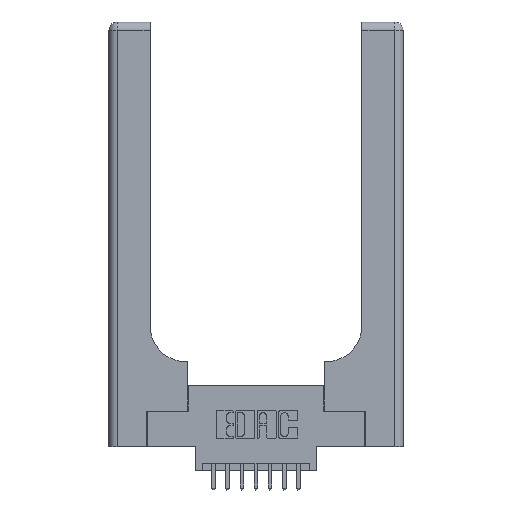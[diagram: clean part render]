
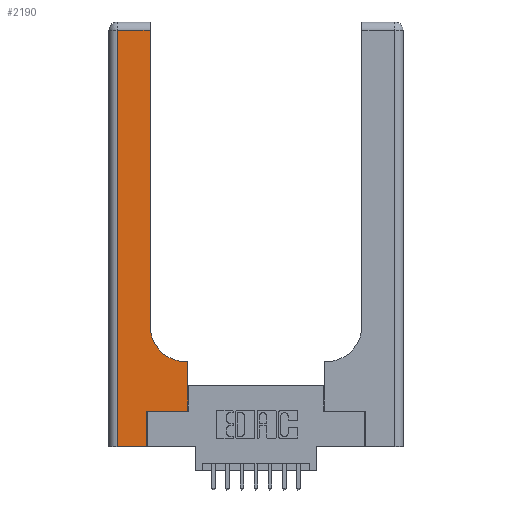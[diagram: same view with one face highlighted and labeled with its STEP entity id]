
A CAD part, top view. The second image highlights one B-rep face of the part: STEP entity #2190.
In plain terms, the highlighted planar face has unit normal (0, 0, 1).
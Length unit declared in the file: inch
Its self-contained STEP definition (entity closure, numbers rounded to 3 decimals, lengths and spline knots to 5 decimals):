
#70 = CARTESIAN_POINT ( 'NONE',  ( 0., 2.94, 0.37 ) ) ;
#260 = EDGE_CURVE ( 'NONE', #14906, #10242, #384, .T. ) ;
#367 = DIRECTION ( 'NONE',  ( -1., 0., 0. ) ) ;
#384 = LINE ( 'NONE', #7655, #14273 ) ;
#699 = CARTESIAN_POINT ( 'NONE',  ( 0.2915, 0.85, 0.37 ) ) ;
#1357 = VERTEX_POINT ( 'NONE', #14289 ) ;
#1389 = DIRECTION ( 'NONE',  ( 1., 0., 0. ) ) ;
#1501 = VERTEX_POINT ( 'NONE', #14553 ) ;
#1813 = DIRECTION ( 'NONE',  ( 0., -1., 0. ) ) ;
#1826 = EDGE_LOOP ( 'NONE', ( #10943, #7124, #8172, #3661, #12264, #11714, #10814, #2758, #12633 ) ) ;
#1890 = VERTEX_POINT ( 'NONE', #3290 ) ;
#2190 = ADVANCED_FACE ( 'NONE', ( #2888 ), #12406, .F. ) ;
#2295 = AXIS2_PLACEMENT_3D ( 'NONE', #10333, #4394, #4304 ) ;
#2758 = ORIENTED_EDGE ( 'NONE', *, *, #260, .T. ) ;
#2888 = FACE_OUTER_BOUND ( 'NONE', #1826, .T. ) ;
#3202 = DIRECTION ( 'NONE',  ( -1., 0., 0. ) ) ;
#3290 = CARTESIAN_POINT ( 'NONE',  ( 0.06, 0., 0.37 ) ) ;
#3437 = VERTEX_POINT ( 'NONE', #9979 ) ;
#3661 = ORIENTED_EDGE ( 'NONE', *, *, #9320, .T. ) ;
#3778 = EDGE_CURVE ( 'NONE', #10242, #10791, #13706, .T. ) ;
#3946 = EDGE_CURVE ( 'NONE', #1501, #14906, #14652, .T. ) ;
#4304 = DIRECTION ( 'NONE',  ( 1., 0., 0. ) ) ;
#4394 = DIRECTION ( 'NONE',  ( 0., 0., -1. ) ) ;
#4674 = LINE ( 'NONE', #9700, #7857 ) ;
#4717 = CARTESIAN_POINT ( 'NONE',  ( 0.5585, 0.6, 0.37 ) ) ;
#4750 = LINE ( 'NONE', #70, #8299 ) ;
#5001 = CARTESIAN_POINT ( 'NONE',  ( 0.269, 0.25, 0.37 ) ) ;
#5084 = CARTESIAN_POINT ( 'NONE',  ( 0.269, 0.25, 0.37 ) ) ;
#5928 = VERTEX_POINT ( 'NONE', #6114 ) ;
#6114 = CARTESIAN_POINT ( 'NONE',  ( 0.2915, 2.94, 0.37 ) ) ;
#6499 = EDGE_CURVE ( 'NONE', #5928, #3437, #4750, .T. ) ;
#6683 = VECTOR ( 'NONE', #14177, 39.37008 ) ;
#6709 = VECTOR ( 'NONE', #1813, 39.37008 ) ;
#6861 = VECTOR ( 'NONE', #12170, 39.37008 ) ;
#7124 = ORIENTED_EDGE ( 'NONE', *, *, #6499, .T. ) ;
#7655 = CARTESIAN_POINT ( 'NONE',  ( 0.2915, 0.6, 0.37 ) ) ;
#7807 = LINE ( 'NONE', #10954, #6861 ) ;
#7857 = VECTOR ( 'NONE', #12146, 39.37008 ) ;
#7888 = EDGE_CURVE ( 'NONE', #1357, #15262, #8619, .T. ) ;
#8172 = ORIENTED_EDGE ( 'NONE', *, *, #10016, .T. ) ;
#8299 = VECTOR ( 'NONE', #13073, 39.37008 ) ;
#8619 = LINE ( 'NONE', #10103, #11353 ) ;
#9311 = VECTOR ( 'NONE', #1389, 39.37008 ) ;
#9320 = EDGE_CURVE ( 'NONE', #1890, #1357, #4674, .T. ) ;
#9700 = CARTESIAN_POINT ( 'NONE',  ( 0., 0., 0.37 ) ) ;
#9979 = CARTESIAN_POINT ( 'NONE',  ( 0.06, 2.94, 0.37 ) ) ;
#10016 = EDGE_CURVE ( 'NONE', #3437, #1890, #13537, .T. ) ;
#10076 = DIRECTION ( 'NONE',  ( 0., 0., -1. ) ) ;
#10103 = CARTESIAN_POINT ( 'NONE',  ( 0.269, 0., 0.37 ) ) ;
#10242 = VERTEX_POINT ( 'NONE', #14617 ) ;
#10333 = CARTESIAN_POINT ( 'NONE',  ( 0.5415, 0.85, 0.37 ) ) ;
#10791 = VERTEX_POINT ( 'NONE', #699 ) ;
#10814 = ORIENTED_EDGE ( 'NONE', *, *, #3946, .T. ) ;
#10943 = ORIENTED_EDGE ( 'NONE', *, *, #15510, .T. ) ;
#10954 = CARTESIAN_POINT ( 'NONE',  ( 0.2915, 3., 0.37 ) ) ;
#11353 = VECTOR ( 'NONE', #14879, 39.37008 ) ;
#11714 = ORIENTED_EDGE ( 'NONE', *, *, #15156, .T. ) ;
#12146 = DIRECTION ( 'NONE',  ( 1., 0., 0. ) ) ;
#12170 = DIRECTION ( 'NONE',  ( 0., 1., 0. ) ) ;
#12264 = ORIENTED_EDGE ( 'NONE', *, *, #7888, .T. ) ;
#12406 = PLANE ( 'NONE',  #13858 ) ;
#12633 = ORIENTED_EDGE ( 'NONE', *, *, #3778, .T. ) ;
#12811 = CARTESIAN_POINT ( 'NONE',  ( 0.06, 3., 0.37 ) ) ;
#12957 = CARTESIAN_POINT ( 'NONE',  ( 0.5585, 0.25, 0.37 ) ) ;
#13073 = DIRECTION ( 'NONE',  ( -1., 0., 0. ) ) ;
#13537 = LINE ( 'NONE', #12811, #6709 ) ;
#13626 = CARTESIAN_POINT ( 'NONE',  ( 0., 3., 0.37 ) ) ;
#13706 = CIRCLE ( 'NONE', #2295, 0.25 ) ;
#13858 = AXIS2_PLACEMENT_3D ( 'NONE', #13626, #10076, #367 ) ;
#14177 = DIRECTION ( 'NONE',  ( 0., 1., 0. ) ) ;
#14273 = VECTOR ( 'NONE', #3202, 39.37008 ) ;
#14289 = CARTESIAN_POINT ( 'NONE',  ( 0.269, 0., 0.37 ) ) ;
#14553 = CARTESIAN_POINT ( 'NONE',  ( 0.5585, 0.25, 0.37 ) ) ;
#14617 = CARTESIAN_POINT ( 'NONE',  ( 0.5415, 0.6, 0.37 ) ) ;
#14652 = LINE ( 'NONE', #12957, #6683 ) ;
#14855 = LINE ( 'NONE', #5084, #9311 ) ;
#14879 = DIRECTION ( 'NONE',  ( 0., 1., 0. ) ) ;
#14906 = VERTEX_POINT ( 'NONE', #4717 ) ;
#15156 = EDGE_CURVE ( 'NONE', #15262, #1501, #14855, .T. ) ;
#15262 = VERTEX_POINT ( 'NONE', #5001 ) ;
#15510 = EDGE_CURVE ( 'NONE', #10791, #5928, #7807, .T. ) ;
